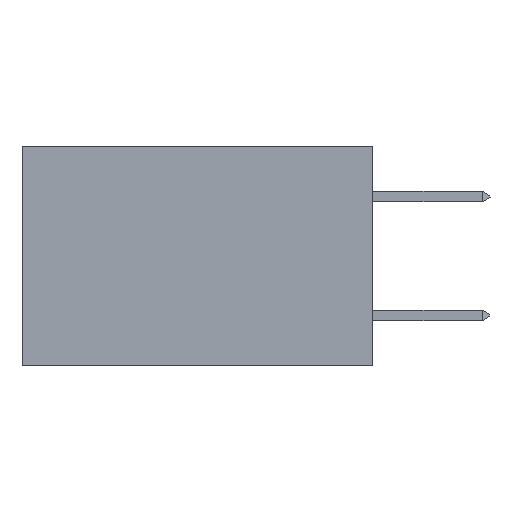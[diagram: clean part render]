
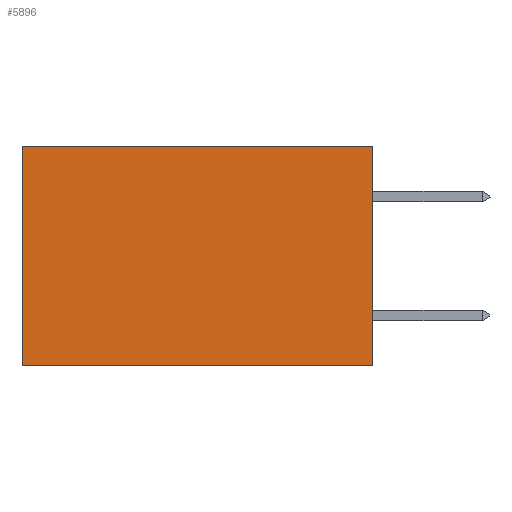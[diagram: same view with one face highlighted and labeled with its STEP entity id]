
A CAD part, left-side view. The second image highlights one B-rep face of the part: STEP entity #5896.
In plain terms, the highlighted planar face has unit normal (-1, 0, 0).
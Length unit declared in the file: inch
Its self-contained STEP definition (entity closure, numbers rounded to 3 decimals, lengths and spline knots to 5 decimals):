
#628 = ORIENTED_EDGE ( 'NONE', *, *, #10514, .F. ) ;
#642 = FACE_OUTER_BOUND ( 'NONE', #12941, .T. ) ;
#702 = CARTESIAN_POINT ( 'NONE',  ( 0.277, 0.59, 0. ) ) ;
#2686 = VERTEX_POINT ( 'NONE', #5992 ) ;
#3678 = ORIENTED_EDGE ( 'NONE', *, *, #6147, .T. ) ;
#3831 = DIRECTION ( 'NONE',  ( 0., 1., 0. ) ) ;
#4297 = ORIENTED_EDGE ( 'NONE', *, *, #11651, .F. ) ;
#4389 = VERTEX_POINT ( 'NONE', #7071 ) ;
#4415 = VERTEX_POINT ( 'NONE', #702 ) ;
#5775 = CARTESIAN_POINT ( 'NONE',  ( 0.277, 0., -0.37 ) ) ;
#5896 = ADVANCED_FACE ( 'NONE', ( #642 ), #10937, .F. ) ;
#5943 = LINE ( 'NONE', #6024, #11130 ) ;
#5977 = DIRECTION ( 'NONE',  ( 0., 0., -1. ) ) ;
#5992 = CARTESIAN_POINT ( 'NONE',  ( 0.277, 0., -0.37 ) ) ;
#6024 = CARTESIAN_POINT ( 'NONE',  ( 0.277, 0.59, -0.37 ) ) ;
#6147 = EDGE_CURVE ( 'NONE', #4415, #11820, #5943, .T. ) ;
#6245 = DIRECTION ( 'NONE',  ( 0., 1., 0. ) ) ;
#6278 = CARTESIAN_POINT ( 'NONE',  ( 0.277, 0., 0. ) ) ;
#6624 = VECTOR ( 'NONE', #13356, 39.37008 ) ;
#7071 = CARTESIAN_POINT ( 'NONE',  ( 0.277, 0., 0. ) ) ;
#7711 = EDGE_CURVE ( 'NONE', #4389, #4415, #9012, .T. ) ;
#7985 = LINE ( 'NONE', #11590, #8369 ) ;
#8369 = VECTOR ( 'NONE', #3831, 39.37008 ) ;
#9012 = LINE ( 'NONE', #6278, #14253 ) ;
#9737 = ORIENTED_EDGE ( 'NONE', *, *, #7711, .T. ) ;
#10174 = AXIS2_PLACEMENT_3D ( 'NONE', #10999, #10911, #10893 ) ;
#10514 = EDGE_CURVE ( 'NONE', #4389, #2686, #14176, .T. ) ;
#10893 = DIRECTION ( 'NONE',  ( 0., 0., -1. ) ) ;
#10911 = DIRECTION ( 'NONE',  ( 1., 0., 0. ) ) ;
#10937 = PLANE ( 'NONE',  #10174 ) ;
#10999 = CARTESIAN_POINT ( 'NONE',  ( 0.277, 0., -0.37 ) ) ;
#11130 = VECTOR ( 'NONE', #5977, 39.37008 ) ;
#11590 = CARTESIAN_POINT ( 'NONE',  ( 0.277, 0., -0.37 ) ) ;
#11651 = EDGE_CURVE ( 'NONE', #2686, #11820, #7985, .T. ) ;
#11820 = VERTEX_POINT ( 'NONE', #13919 ) ;
#12941 = EDGE_LOOP ( 'NONE', ( #3678, #4297, #628, #9737 ) ) ;
#13356 = DIRECTION ( 'NONE',  ( 0., 0., -1. ) ) ;
#13919 = CARTESIAN_POINT ( 'NONE',  ( 0.277, 0.59, -0.37 ) ) ;
#14176 = LINE ( 'NONE', #5775, #6624 ) ;
#14253 = VECTOR ( 'NONE', #6245, 39.37008 ) ;
